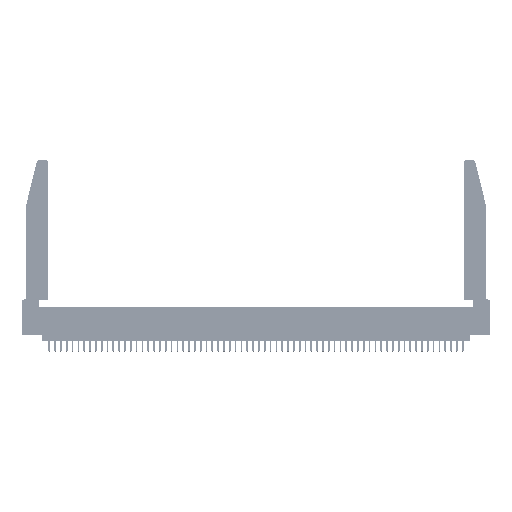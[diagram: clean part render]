
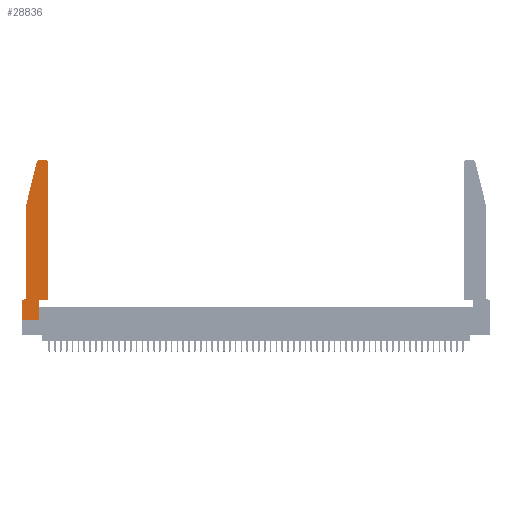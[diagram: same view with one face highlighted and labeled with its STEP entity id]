
A CAD part, top view. The second image highlights one B-rep face of the part: STEP entity #28836.
In plain terms, the highlighted planar face has unit normal (0, 0, 1).
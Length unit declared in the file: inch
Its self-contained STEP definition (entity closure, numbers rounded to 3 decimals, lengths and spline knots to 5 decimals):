
#425 = CARTESIAN_POINT ( 'NONE',  ( 0.2865, 0.35, 0.37 ) ) ;
#1262 = DIRECTION ( 'NONE',  ( 0., 0., -1. ) ) ;
#1263 = CARTESIAN_POINT ( 'NONE',  ( 0.284, 2.72, 0.37 ) ) ;
#2550 = CARTESIAN_POINT ( 'NONE',  ( 0.0755, 2., 0.37 ) ) ;
#3743 = EDGE_CURVE ( 'NONE', #9976, #17677, #41878, .T. ) ;
#3906 = EDGE_CURVE ( 'NONE', #17898, #27852, #43928, .T. ) ;
#4327 = DIRECTION ( 'NONE',  ( 1., 0., 0. ) ) ;
#5458 = VECTOR ( 'NONE', #11541, 39.37008 ) ;
#5789 = DIRECTION ( 'NONE',  ( 1., 0., 0. ) ) ;
#6650 = VECTOR ( 'NONE', #15642, 39.37008 ) ;
#7026 = CARTESIAN_POINT ( 'NONE',  ( 0.4505, 0.35, 0.37 ) ) ;
#9076 = DIRECTION ( 'NONE',  ( 0., 1., 0. ) ) ;
#9297 = FACE_OUTER_BOUND ( 'NONE', #27011, .T. ) ;
#9976 = VERTEX_POINT ( 'NONE', #10083 ) ;
#10083 = CARTESIAN_POINT ( 'NONE',  ( 0.0755, 0.42, 0.37 ) ) ;
#11541 = DIRECTION ( 'NONE',  ( 0., 1., 0. ) ) ;
#11945 = ORIENTED_EDGE ( 'NONE', *, *, #27672, .T. ) ;
#12024 = CARTESIAN_POINT ( 'NONE',  ( 0., 0.35, 0.37 ) ) ;
#12679 = EDGE_CURVE ( 'NONE', #28651, #43761, #50211, .T. ) ;
#13266 = LINE ( 'NONE', #2550, #31298 ) ;
#15642 = DIRECTION ( 'NONE',  ( -1., 0., 0. ) ) ;
#15809 = CARTESIAN_POINT ( 'NONE',  ( 0.4205, 2.72, 0.37 ) ) ;
#16380 = VECTOR ( 'NONE', #9076, 39.37008 ) ;
#16498 = DIRECTION ( 'NONE',  ( 1., 0., 0. ) ) ;
#16743 = ORIENTED_EDGE ( 'NONE', *, *, #42113, .T. ) ;
#17677 = VERTEX_POINT ( 'NONE', #44325 ) ;
#17898 = VERTEX_POINT ( 'NONE', #54494 ) ;
#18025 = CARTESIAN_POINT ( 'NONE',  ( 0.4505, 0.35, 0.37 ) ) ;
#18493 = AXIS2_PLACEMENT_3D ( 'NONE', #12024, #43003, #16498 ) ;
#19347 = DIRECTION ( 'NONE',  ( 1., 0., 0. ) ) ;
#19880 = AXIS2_PLACEMENT_3D ( 'NONE', #1263, #32421, #5789 ) ;
#20307 = DIRECTION ( 'NONE',  ( 1., 0., 0. ) ) ;
#20474 = VERTEX_POINT ( 'NONE', #44677 ) ;
#24529 = ORIENTED_EDGE ( 'NONE', *, *, #12679, .T. ) ;
#24738 = DIRECTION ( 'NONE',  ( -1., 0., 0. ) ) ;
#26127 = VERTEX_POINT ( 'NONE', #46390 ) ;
#26400 = AXIS2_PLACEMENT_3D ( 'NONE', #28012, #1262, #32420 ) ;
#26758 = CARTESIAN_POINT ( 'NONE',  ( 0.25487, 2.72718, 0.37 ) ) ;
#26967 = ORIENTED_EDGE ( 'NONE', *, *, #27549, .T. ) ;
#27011 = EDGE_LOOP ( 'NONE', ( #46252, #54000, #44187, #11945, #49197, #26967, #31450, #28713, #24529, #46604, #16743, #42547 ) ) ;
#27549 = EDGE_CURVE ( 'NONE', #17677, #30794, #53758, .T. ) ;
#27672 = EDGE_CURVE ( 'NONE', #20474, #9976, #44113, .T. ) ;
#27852 = VERTEX_POINT ( 'NONE', #40017 ) ;
#28012 = CARTESIAN_POINT ( 'NONE',  ( 0.0055, 0.42, 0.37 ) ) ;
#28651 = VERTEX_POINT ( 'NONE', #45894 ) ;
#28713 = ORIENTED_EDGE ( 'NONE', *, *, #32438, .T. ) ;
#28836 = ADVANCED_FACE ( 'NONE', ( #9297 ), #56130, .T. ) ;
#29418 = CIRCLE ( 'NONE', #19880, 0.03 ) ;
#29541 = CIRCLE ( 'NONE', #31053, 0.03 ) ;
#30794 = VERTEX_POINT ( 'NONE', #34187 ) ;
#31053 = AXIS2_PLACEMENT_3D ( 'NONE', #15809, #46752, #20307 ) ;
#31298 = VECTOR ( 'NONE', #46981, 39.37008 ) ;
#31450 = ORIENTED_EDGE ( 'NONE', *, *, #37873, .T. ) ;
#31714 = CARTESIAN_POINT ( 'NONE',  ( 0., 0., 0.37 ) ) ;
#31887 = VECTOR ( 'NONE', #4327, 39.37008 ) ;
#32158 = VECTOR ( 'NONE', #24738, 39.37008 ) ;
#32355 = VECTOR ( 'NONE', #34250, 39.37008 ) ;
#32420 = DIRECTION ( 'NONE',  ( -1., 0., 0. ) ) ;
#32421 = DIRECTION ( 'NONE',  ( 0., 0., 1. ) ) ;
#32438 = EDGE_CURVE ( 'NONE', #26127, #28651, #33302, .T. ) ;
#32677 = EDGE_CURVE ( 'NONE', #43761, #50807, #56049, .T. ) ;
#32996 = LINE ( 'NONE', #31714, #41963 ) ;
#33302 = LINE ( 'NONE', #39882, #31887 ) ;
#34187 = CARTESIAN_POINT ( 'NONE',  ( 0., 0.35, 0.37 ) ) ;
#34250 = DIRECTION ( 'NONE',  ( 0., -1., 0. ) ) ;
#36016 = EDGE_CURVE ( 'NONE', #27852, #46150, #29418, .T. ) ;
#37873 = EDGE_CURVE ( 'NONE', #30794, #26127, #32996, .T. ) ;
#38138 = EDGE_CURVE ( 'NONE', #47635, #17898, #29541, .T. ) ;
#39882 = CARTESIAN_POINT ( 'NONE',  ( 0., 0., 0.37 ) ) ;
#40017 = CARTESIAN_POINT ( 'NONE',  ( 0.284, 2.75, 0.37 ) ) ;
#41385 = CARTESIAN_POINT ( 'NONE',  ( 0.4505, 0.35, 0.37 ) ) ;
#41878 = CIRCLE ( 'NONE', #26400, 0.07 ) ;
#41963 = VECTOR ( 'NONE', #53871, 39.37008 ) ;
#42113 = EDGE_CURVE ( 'NONE', #50807, #47635, #51215, .T. ) ;
#42272 = CARTESIAN_POINT ( 'NONE',  ( 0.2605, 2.75, 0.37 ) ) ;
#42547 = ORIENTED_EDGE ( 'NONE', *, *, #38138, .T. ) ;
#42926 = VECTOR ( 'NONE', #19347, 39.37008 ) ;
#43003 = DIRECTION ( 'NONE',  ( 0., 0., 1. ) ) ;
#43620 = CARTESIAN_POINT ( 'NONE',  ( 0.4505, 2.72, 0.37 ) ) ;
#43761 = VERTEX_POINT ( 'NONE', #425 ) ;
#43928 = LINE ( 'NONE', #42272, #32158 ) ;
#44113 = LINE ( 'NONE', #47360, #32355 ) ;
#44187 = ORIENTED_EDGE ( 'NONE', *, *, #46833, .T. ) ;
#44325 = CARTESIAN_POINT ( 'NONE',  ( 0.0055, 0.35, 0.37 ) ) ;
#44546 = CARTESIAN_POINT ( 'NONE',  ( 0.2865, 0.35, 0.37 ) ) ;
#44677 = CARTESIAN_POINT ( 'NONE',  ( 0.0755, 2., 0.37 ) ) ;
#45894 = CARTESIAN_POINT ( 'NONE',  ( 0.2865, 0., 0.37 ) ) ;
#46150 = VERTEX_POINT ( 'NONE', #26758 ) ;
#46252 = ORIENTED_EDGE ( 'NONE', *, *, #3906, .T. ) ;
#46390 = CARTESIAN_POINT ( 'NONE',  ( 0., 0., 0.37 ) ) ;
#46604 = ORIENTED_EDGE ( 'NONE', *, *, #32677, .T. ) ;
#46752 = DIRECTION ( 'NONE',  ( 0., 0., 1. ) ) ;
#46833 = EDGE_CURVE ( 'NONE', #46150, #20474, #13266, .T. ) ;
#46981 = DIRECTION ( 'NONE',  ( -0.239, -0.971, 0. ) ) ;
#47360 = CARTESIAN_POINT ( 'NONE',  ( 0.0755, 2., 0.37 ) ) ;
#47635 = VERTEX_POINT ( 'NONE', #43620 ) ;
#49197 = ORIENTED_EDGE ( 'NONE', *, *, #3743, .T. ) ;
#50211 = LINE ( 'NONE', #44546, #16380 ) ;
#50807 = VERTEX_POINT ( 'NONE', #18025 ) ;
#51215 = LINE ( 'NONE', #7026, #5458 ) ;
#53758 = LINE ( 'NONE', #55464, #6650 ) ;
#53871 = DIRECTION ( 'NONE',  ( 0., -1., 0. ) ) ;
#54000 = ORIENTED_EDGE ( 'NONE', *, *, #36016, .T. ) ;
#54494 = CARTESIAN_POINT ( 'NONE',  ( 0.4205, 2.75, 0.37 ) ) ;
#55464 = CARTESIAN_POINT ( 'NONE',  ( 0.0755, 0.35, 0.37 ) ) ;
#56049 = LINE ( 'NONE', #41385, #42926 ) ;
#56130 = PLANE ( 'NONE',  #18493 ) ;
